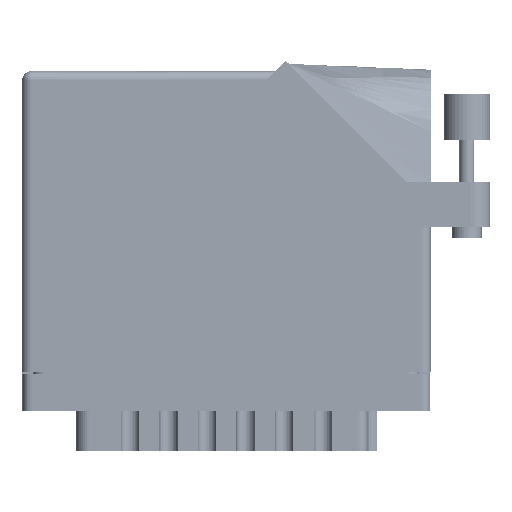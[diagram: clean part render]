
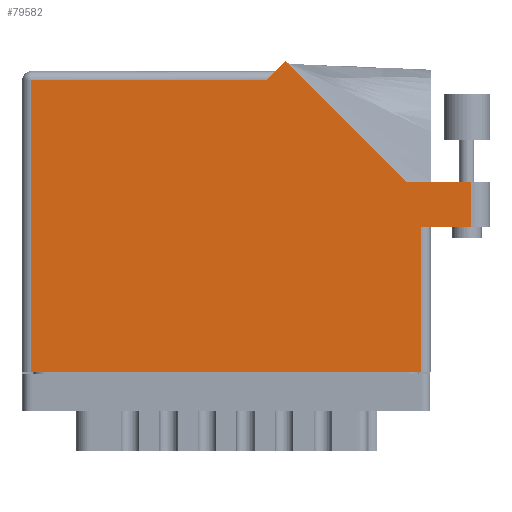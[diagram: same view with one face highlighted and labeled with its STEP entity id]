
A CAD part, front view. The second image highlights one B-rep face of the part: STEP entity #79582.
In plain terms, the highlighted face is planar.
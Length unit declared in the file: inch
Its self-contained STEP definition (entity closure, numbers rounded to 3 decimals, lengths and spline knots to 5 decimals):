
#801 = CARTESIAN_POINT ( 'NONE',  ( 3.155, 1.287, 0. ) ) ;
#3513 = CARTESIAN_POINT ( 'NONE',  ( 2.58942, 1.287, 0. ) ) ;
#3764 = ORIENTED_EDGE ( 'NONE', *, *, #27341, .T. ) ;
#5421 = VECTOR ( 'NONE', #70193, 39.37008 ) ;
#5815 = VECTOR ( 'NONE', #83752, 39.37008 ) ;
#5844 = ORIENTED_EDGE ( 'NONE', *, *, #79068, .T. ) ;
#11431 = EDGE_CURVE ( 'NONE', #47591, #40468, #60440, .T. ) ;
#12848 = VERTEX_POINT ( 'NONE', #23736 ) ;
#13084 = LINE ( 'NONE', #33778, #86085 ) ;
#14936 = EDGE_CURVE ( 'NONE', #12848, #73335, #40652, .T. ) ;
#15101 = DIRECTION ( 'NONE',  ( -0.707, -0.707, 0. ) ) ;
#16633 = DIRECTION ( 'NONE',  ( 0., -1., 0. ) ) ;
#17879 = CARTESIAN_POINT ( 'NONE',  ( 3.03, 1.287, 0. ) ) ;
#20926 = EDGE_CURVE ( 'NONE', #40468, #12848, #45316, .T. ) ;
#21409 = LINE ( 'NONE', #47881, #52903 ) ;
#22859 = ORIENTED_EDGE ( 'NONE', *, *, #69971, .T. ) ;
#23736 = CARTESIAN_POINT ( 'NONE',  ( 1.643, 1.968, 0. ) ) ;
#23982 = FACE_OUTER_BOUND ( 'NONE', #37511, .T. ) ;
#25176 = VERTEX_POINT ( 'NONE', #32301 ) ;
#26036 = AXIS2_PLACEMENT_3D ( 'NONE', #49688, #43357, #64156 ) ;
#27341 = EDGE_CURVE ( 'NONE', #82663, #46851, #83391, .T. ) ;
#32301 = CARTESIAN_POINT ( 'NONE',  ( 0.062, 0., 0. ) ) ;
#32830 = ORIENTED_EDGE ( 'NONE', *, *, #90799, .T. ) ;
#33064 = DIRECTION ( 'NONE',  ( 1., 0., 0. ) ) ;
#33778 = CARTESIAN_POINT ( 'NONE',  ( 0., 0., 0. ) ) ;
#35726 = CARTESIAN_POINT ( 'NONE',  ( 0.062, 1.968, 0. ) ) ;
#35895 = DIRECTION ( 'NONE',  ( -1., 0., 0. ) ) ;
#37511 = EDGE_LOOP ( 'NONE', ( #32830, #82426, #5844, #74602, #64428, #55675, #86931, #22859, #3764 ) ) ;
#38613 = VECTOR ( 'NONE', #46499, 39.37008 ) ;
#40468 = VERTEX_POINT ( 'NONE', #43638 ) ;
#40652 = LINE ( 'NONE', #77174, #5815 ) ;
#43357 = DIRECTION ( 'NONE',  ( 0., 0., -1. ) ) ;
#43638 = CARTESIAN_POINT ( 'NONE',  ( 1.77571, 2.10071, 0. ) ) ;
#45316 = LINE ( 'NONE', #92921, #53153 ) ;
#46499 = DIRECTION ( 'NONE',  ( 0., 1., 0. ) ) ;
#46851 = VERTEX_POINT ( 'NONE', #65501 ) ;
#47591 = VERTEX_POINT ( 'NONE', #3513 ) ;
#47881 = CARTESIAN_POINT ( 'NONE',  ( 2.755, 0.98, 0. ) ) ;
#48746 = EDGE_CURVE ( 'NONE', #61465, #55153, #79114, .T. ) ;
#49688 = CARTESIAN_POINT ( 'NONE',  ( 0., 2.03, 0. ) ) ;
#52903 = VECTOR ( 'NONE', #33064, 39.37008 ) ;
#53153 = VECTOR ( 'NONE', #15101, 39.37008 ) ;
#53401 = VECTOR ( 'NONE', #35895, 39.37008 ) ;
#55073 = EDGE_CURVE ( 'NONE', #73335, #25176, #81810, .T. ) ;
#55153 = VERTEX_POINT ( 'NONE', #17879 ) ;
#55675 = ORIENTED_EDGE ( 'NONE', *, *, #14936, .T. ) ;
#58475 = DIRECTION ( 'NONE',  ( 0., 1., 0. ) ) ;
#60440 = LINE ( 'NONE', #62957, #5421 ) ;
#61465 = VERTEX_POINT ( 'NONE', #74965 ) ;
#62568 = PLANE ( 'NONE',  #26036 ) ;
#62957 = CARTESIAN_POINT ( 'NONE',  ( 2.58942, 1.287, 0. ) ) ;
#64156 = DIRECTION ( 'NONE',  ( -1., 0., 0. ) ) ;
#64428 = ORIENTED_EDGE ( 'NONE', *, *, #20926, .T. ) ;
#65501 = CARTESIAN_POINT ( 'NONE',  ( 2.693, 0.98, 0. ) ) ;
#69045 = DIRECTION ( 'NONE',  ( 1., 0., 0. ) ) ;
#69971 = EDGE_CURVE ( 'NONE', #25176, #82663, #13084, .T. ) ;
#70193 = DIRECTION ( 'NONE',  ( -0.707, 0.707, 0. ) ) ;
#73335 = VERTEX_POINT ( 'NONE', #35726 ) ;
#74602 = ORIENTED_EDGE ( 'NONE', *, *, #11431, .T. ) ;
#74965 = CARTESIAN_POINT ( 'NONE',  ( 3.03, 0.98, 0. ) ) ;
#75431 = CARTESIAN_POINT ( 'NONE',  ( 2.693, 0., 0. ) ) ;
#77174 = CARTESIAN_POINT ( 'NONE',  ( 0., 1.968, 0. ) ) ;
#79068 = EDGE_CURVE ( 'NONE', #55153, #47591, #91550, .T. ) ;
#79114 = LINE ( 'NONE', #82271, #38613 ) ;
#79582 = ADVANCED_FACE ( 'NONE', ( #23982 ), #62568, .F. ) ;
#81066 = VECTOR ( 'NONE', #58475, 39.37008 ) ;
#81810 = LINE ( 'NONE', #82255, #87399 ) ;
#82255 = CARTESIAN_POINT ( 'NONE',  ( 0.062, 0., 0. ) ) ;
#82271 = CARTESIAN_POINT ( 'NONE',  ( 3.03, 1.287, 0. ) ) ;
#82426 = ORIENTED_EDGE ( 'NONE', *, *, #48746, .T. ) ;
#82663 = VERTEX_POINT ( 'NONE', #75431 ) ;
#83391 = LINE ( 'NONE', #88277, #81066 ) ;
#83752 = DIRECTION ( 'NONE',  ( -1., 0., 0. ) ) ;
#86085 = VECTOR ( 'NONE', #69045, 39.37008 ) ;
#86931 = ORIENTED_EDGE ( 'NONE', *, *, #55073, .T. ) ;
#87399 = VECTOR ( 'NONE', #16633, 39.37008 ) ;
#88277 = CARTESIAN_POINT ( 'NONE',  ( 2.693, 0.98, 0. ) ) ;
#90799 = EDGE_CURVE ( 'NONE', #46851, #61465, #21409, .T. ) ;
#91550 = LINE ( 'NONE', #801, #53401 ) ;
#92921 = CARTESIAN_POINT ( 'NONE',  ( 1.705, 2.03, 0. ) ) ;
